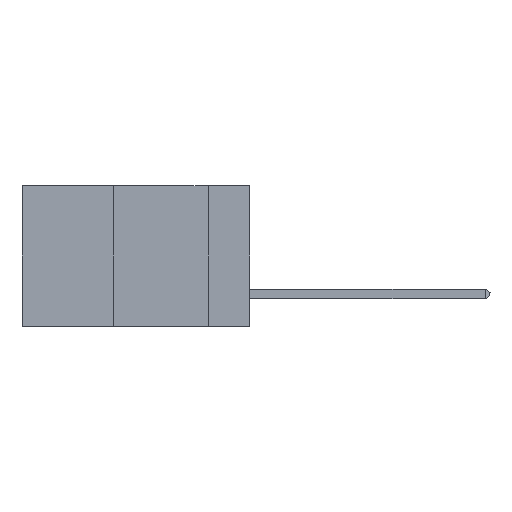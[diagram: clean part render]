
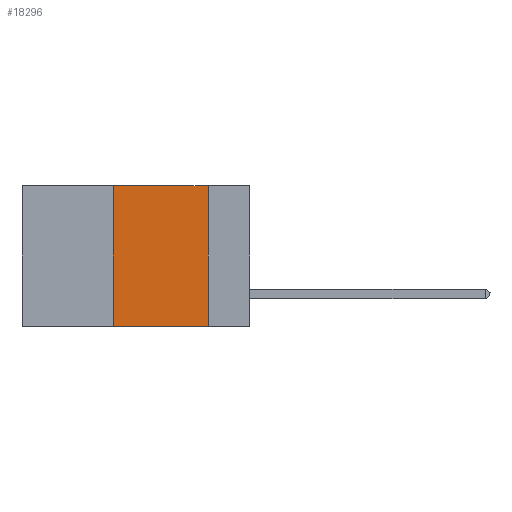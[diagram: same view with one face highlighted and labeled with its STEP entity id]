
A CAD part, left-side view. The second image highlights one B-rep face of the part: STEP entity #18296.
In plain terms, the highlighted planar face has unit normal (-1, 0, 0).
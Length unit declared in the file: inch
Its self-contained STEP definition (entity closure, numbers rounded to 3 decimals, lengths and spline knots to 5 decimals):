
#1092 = LINE ( 'NONE', #26068, #27904 ) ;
#2191 = ORIENTED_EDGE ( 'NONE', *, *, #6284, .T. ) ;
#3781 = ORIENTED_EDGE ( 'NONE', *, *, #27289, .F. ) ;
#5386 = CARTESIAN_POINT ( 'NONE',  ( 0., 0.36, -0.37 ) ) ;
#5968 = LINE ( 'NONE', #15250, #8547 ) ;
#6284 = EDGE_CURVE ( 'NONE', #19057, #9989, #25450, .T. ) ;
#6360 = VECTOR ( 'NONE', #25967, 39.37008 ) ;
#6531 = LINE ( 'NONE', #20487, #16077 ) ;
#8547 = VECTOR ( 'NONE', #17613, 39.37008 ) ;
#8730 = ORIENTED_EDGE ( 'NONE', *, *, #14342, .F. ) ;
#9989 = VERTEX_POINT ( 'NONE', #28185 ) ;
#12216 = DIRECTION ( 'NONE',  ( 1., 0., 0. ) ) ;
#12702 = CARTESIAN_POINT ( 'NONE',  ( 0., 0.11, 0. ) ) ;
#14342 = EDGE_CURVE ( 'NONE', #19892, #14494, #6531, .T. ) ;
#14494 = VERTEX_POINT ( 'NONE', #12702 ) ;
#15250 = CARTESIAN_POINT ( 'NONE',  ( 0., 0.36, 0. ) ) ;
#16036 = EDGE_LOOP ( 'NONE', ( #3781, #8730, #30489, #2191 ) ) ;
#16077 = VECTOR ( 'NONE', #29498, 39.37008 ) ;
#17613 = DIRECTION ( 'NONE',  ( 0., 0., 1. ) ) ;
#18296 = ADVANCED_FACE ( 'NONE', ( #25702 ), #26317, .F. ) ;
#18463 = CARTESIAN_POINT ( 'NONE',  ( 0., 0.36, 0. ) ) ;
#18729 = EDGE_CURVE ( 'NONE', #19057, #19892, #5968, .T. ) ;
#19057 = VERTEX_POINT ( 'NONE', #5386 ) ;
#19892 = VERTEX_POINT ( 'NONE', #18463 ) ;
#20487 = CARTESIAN_POINT ( 'NONE',  ( 0., 0.6, 0. ) ) ;
#23771 = DIRECTION ( 'NONE',  ( 0., 0., -1. ) ) ;
#25450 = LINE ( 'NONE', #28460, #6360 ) ;
#25702 = FACE_OUTER_BOUND ( 'NONE', #16036, .T. ) ;
#25967 = DIRECTION ( 'NONE',  ( 0., -1., 0. ) ) ;
#26068 = CARTESIAN_POINT ( 'NONE',  ( 0., 0.11, 0. ) ) ;
#26317 = PLANE ( 'NONE',  #28447 ) ;
#27289 = EDGE_CURVE ( 'NONE', #14494, #9989, #1092, .T. ) ;
#27904 = VECTOR ( 'NONE', #28564, 39.37008 ) ;
#28185 = CARTESIAN_POINT ( 'NONE',  ( 0., 0.11, -0.37 ) ) ;
#28447 = AXIS2_PLACEMENT_3D ( 'NONE', #28725, #12216, #23771 ) ;
#28460 = CARTESIAN_POINT ( 'NONE',  ( 0., 0.6, -0.37 ) ) ;
#28564 = DIRECTION ( 'NONE',  ( 0., 0., -1. ) ) ;
#28725 = CARTESIAN_POINT ( 'NONE',  ( 0., 0.6, 0. ) ) ;
#29498 = DIRECTION ( 'NONE',  ( 0., -1., 0. ) ) ;
#30489 = ORIENTED_EDGE ( 'NONE', *, *, #18729, .F. ) ;
